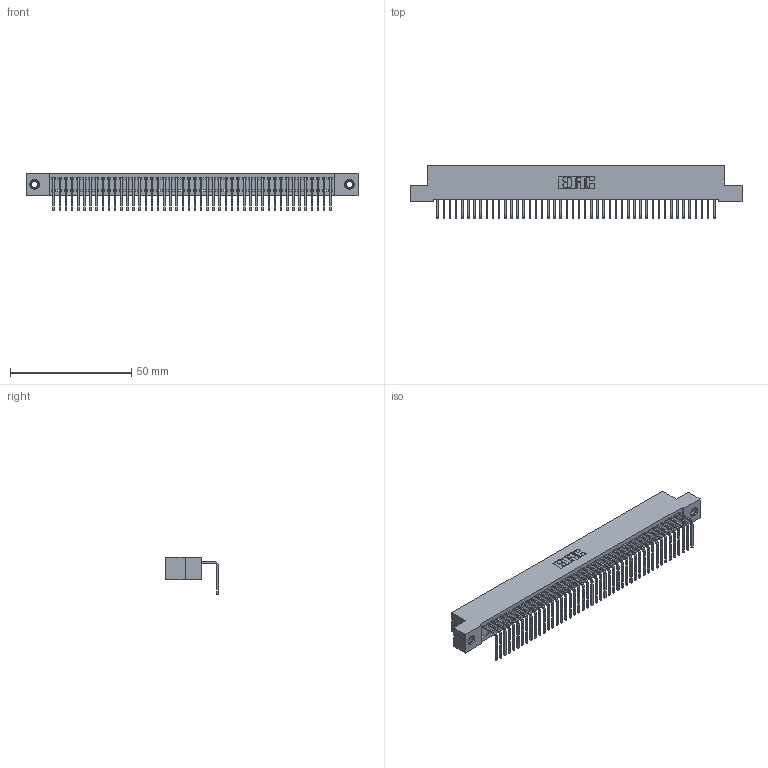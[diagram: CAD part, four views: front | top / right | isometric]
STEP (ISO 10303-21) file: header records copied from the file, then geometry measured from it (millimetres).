
FILE_DESCRIPTION (( 'STEP AP203' ), '1' );
FILE_NAME ('342-046-558-107.STEP', '2018-08-12T16:36:48', ( '' ), ( '' ), 'SwSTEP 2.0', 'SolidWorks 2016', '' );
FILE_SCHEMA (( 'CONFIG_CONTROL_DESIGN' ));
Length unit declared in the file: inch
Products named in the file (4): 345-292-001_558 Tail - 2; 345-250-001_345-250-005-103; 342-046-558-107; 342 Part_TI
Assembly tree (49 placements, depth 2):
  342-046-558-107
    342 Part_TI
    345-292-001_558 Tail - 2  x46
    345-250-001_345-250-005-103  x2
Bounding box: 137.16 x 21.91 x 15.62 mm (x, y, z)
Volume: 12181.5 mm3; surface area: 18865.3 mm2
Topology: 49 solids, 49 shells, 2930 faces, 8807 edges, 5802 vertices
Faces by surface type: plane 2122, cylinder 792, cone 12, torus 4
Entity records: 28742 total; most frequent: CARTESIAN_POINT 4939, ORIENTED_EDGE 4914, DIRECTION 4191, EDGE_CURVE 2457, VECTOR 2309, LINE 2309, VERTEX_POINT 1632, AXIS2_PLACEMENT_3D 941
